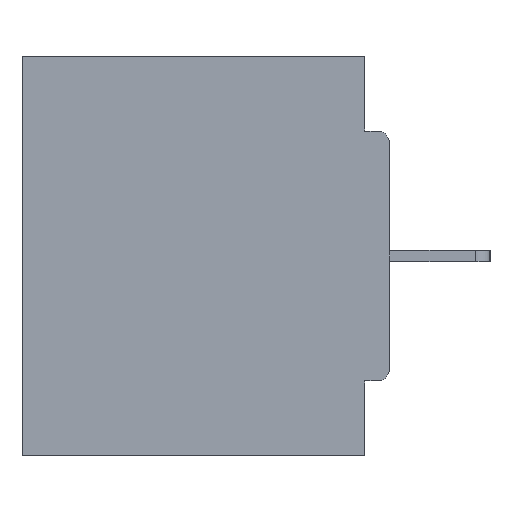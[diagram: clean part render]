
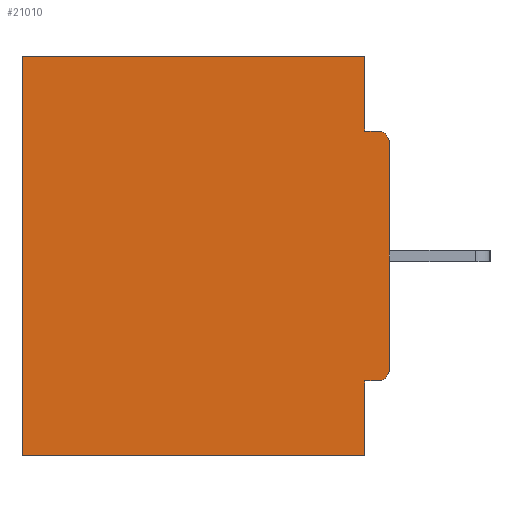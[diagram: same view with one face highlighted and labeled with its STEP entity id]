
A CAD part, left-side view. The second image highlights one B-rep face of the part: STEP entity #21010.
In plain terms, the highlighted planar face has unit normal (-1, 0, 0).
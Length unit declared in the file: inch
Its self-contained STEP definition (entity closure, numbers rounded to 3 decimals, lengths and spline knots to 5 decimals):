
#112 = VERTEX_POINT ( 'NONE', #14981 ) ;
#173 = ORIENTED_EDGE ( 'NONE', *, *, #13140, .F. ) ;
#567 = CARTESIAN_POINT ( 'NONE',  ( 0.298, 0.015, -0.0935 ) ) ;
#664 = VERTEX_POINT ( 'NONE', #13130 ) ;
#939 = EDGE_CURVE ( 'NONE', #664, #19759, #7482, .T. ) ;
#2488 = CARTESIAN_POINT ( 'NONE',  ( 0.298, 0., -0.0935 ) ) ;
#3073 = EDGE_CURVE ( 'NONE', #112, #14863, #17425, .T. ) ;
#3423 = DIRECTION ( 'NONE',  ( 0., 0., -1. ) ) ;
#4201 = VECTOR ( 'NONE', #13381, 39.37008 ) ;
#5898 = DIRECTION ( 'NONE',  ( 1., 0., 0. ) ) ;
#6306 = VERTEX_POINT ( 'NONE', #20187 ) ;
#6440 = CARTESIAN_POINT ( 'NONE',  ( 0.298, 0.015, -0.3915 ) ) ;
#6796 = DIRECTION ( 'NONE',  ( -1., 0., 0. ) ) ;
#7477 = AXIS2_PLACEMENT_3D ( 'NONE', #13451, #5898, #3423 ) ;
#7482 = LINE ( 'NONE', #27811, #12772 ) ;
#7650 = CARTESIAN_POINT ( 'NONE',  ( 0.298, 0.031, -0.5 ) ) ;
#7891 = DIRECTION ( 'NONE',  ( 0., 0., -1. ) ) ;
#8072 = LINE ( 'NONE', #2488, #15989 ) ;
#8828 = LINE ( 'NONE', #21455, #9953 ) ;
#9593 = EDGE_LOOP ( 'NONE', ( #16225, #32142, #21079, #19438, #29886, #173, #20198, #16989, #21119, #31438 ) ) ;
#9953 = VECTOR ( 'NONE', #26861, 39.37008 ) ;
#10351 = CIRCLE ( 'NONE', #22405, 0.015 ) ;
#10411 = CARTESIAN_POINT ( 'NONE',  ( 0.298, 0., 0. ) ) ;
#11147 = PLANE ( 'NONE',  #7477 ) ;
#11295 = LINE ( 'NONE', #28990, #22964 ) ;
#11372 = DIRECTION ( 'NONE',  ( -1., 0., 0. ) ) ;
#11869 = CARTESIAN_POINT ( 'NONE',  ( 0.298, 0., -0.1085 ) ) ;
#11960 = EDGE_CURVE ( 'NONE', #6306, #21548, #8828, .T. ) ;
#12712 = DIRECTION ( 'NONE',  ( 0., 0., -1. ) ) ;
#12772 = VECTOR ( 'NONE', #15191, 39.37008 ) ;
#12986 = VERTEX_POINT ( 'NONE', #7650 ) ;
#13065 = VERTEX_POINT ( 'NONE', #28127 ) ;
#13130 = CARTESIAN_POINT ( 'NONE',  ( 0.298, 0.031, 0. ) ) ;
#13140 = EDGE_CURVE ( 'NONE', #12986, #14863, #26141, .T. ) ;
#13381 = DIRECTION ( 'NONE',  ( 0., 1., 0. ) ) ;
#13451 = CARTESIAN_POINT ( 'NONE',  ( 0.298, 0., 0. ) ) ;
#13645 = LINE ( 'NONE', #28077, #25780 ) ;
#14366 = CARTESIAN_POINT ( 'NONE',  ( 0.298, 0.031, -0.4065 ) ) ;
#14863 = VERTEX_POINT ( 'NONE', #18270 ) ;
#14981 = CARTESIAN_POINT ( 'NONE',  ( 0.298, 0.46, 0. ) ) ;
#15191 = DIRECTION ( 'NONE',  ( 0., 0., -1. ) ) ;
#15989 = VECTOR ( 'NONE', #22844, 39.37008 ) ;
#16216 = DIRECTION ( 'NONE',  ( 0., 1., 0. ) ) ;
#16225 = ORIENTED_EDGE ( 'NONE', *, *, #29226, .T. ) ;
#16989 = ORIENTED_EDGE ( 'NONE', *, *, #11960, .F. ) ;
#17106 = AXIS2_PLACEMENT_3D ( 'NONE', #6440, #11372, #21368 ) ;
#17425 = LINE ( 'NONE', #27250, #18306 ) ;
#18270 = CARTESIAN_POINT ( 'NONE',  ( 0.298, 0.46, -0.5 ) ) ;
#18306 = VECTOR ( 'NONE', #7891, 39.37008 ) ;
#18346 = DIRECTION ( 'NONE',  ( 0., 0., -1. ) ) ;
#18780 = CARTESIAN_POINT ( 'NONE',  ( 0.298, 0., -0.5 ) ) ;
#19438 = ORIENTED_EDGE ( 'NONE', *, *, #31608, .T. ) ;
#19759 = VERTEX_POINT ( 'NONE', #29780 ) ;
#20187 = CARTESIAN_POINT ( 'NONE',  ( 0.298, 0.015, -0.4065 ) ) ;
#20198 = ORIENTED_EDGE ( 'NONE', *, *, #20636, .F. ) ;
#20636 = EDGE_CURVE ( 'NONE', #21548, #12986, #13645, .T. ) ;
#20678 = FACE_OUTER_BOUND ( 'NONE', #9593, .T. ) ;
#21010 = ADVANCED_FACE ( 'NONE', ( #20678 ), #11147, .F. ) ;
#21079 = ORIENTED_EDGE ( 'NONE', *, *, #939, .F. ) ;
#21119 = ORIENTED_EDGE ( 'NONE', *, *, #25135, .T. ) ;
#21368 = DIRECTION ( 'NONE',  ( 0., 0., -1. ) ) ;
#21455 = CARTESIAN_POINT ( 'NONE',  ( 0.298, 0., -0.4065 ) ) ;
#21548 = VERTEX_POINT ( 'NONE', #14366 ) ;
#21701 = VECTOR ( 'NONE', #12712, 39.37008 ) ;
#21885 = CARTESIAN_POINT ( 'NONE',  ( 0.298, 0.015, -0.1085 ) ) ;
#22078 = VERTEX_POINT ( 'NONE', #11869 ) ;
#22333 = CIRCLE ( 'NONE', #17106, 0.015 ) ;
#22405 = AXIS2_PLACEMENT_3D ( 'NONE', #21885, #6796, #18346 ) ;
#22844 = DIRECTION ( 'NONE',  ( 0., -1., 0. ) ) ;
#22964 = VECTOR ( 'NONE', #16216, 39.37008 ) ;
#23172 = DIRECTION ( 'NONE',  ( 0., 0., -1. ) ) ;
#25135 = EDGE_CURVE ( 'NONE', #6306, #13065, #22333, .T. ) ;
#25780 = VECTOR ( 'NONE', #23172, 39.37008 ) ;
#26141 = LINE ( 'NONE', #18780, #4201 ) ;
#26163 = EDGE_CURVE ( 'NONE', #22078, #13065, #30737, .T. ) ;
#26564 = EDGE_CURVE ( 'NONE', #19759, #27559, #8072, .T. ) ;
#26861 = DIRECTION ( 'NONE',  ( 0., 1., 0. ) ) ;
#27250 = CARTESIAN_POINT ( 'NONE',  ( 0.298, 0.46, 0. ) ) ;
#27559 = VERTEX_POINT ( 'NONE', #567 ) ;
#27811 = CARTESIAN_POINT ( 'NONE',  ( 0.298, 0.031, -0.5 ) ) ;
#28077 = CARTESIAN_POINT ( 'NONE',  ( 0.298, 0.031, -0.5 ) ) ;
#28127 = CARTESIAN_POINT ( 'NONE',  ( 0.298, 0., -0.3915 ) ) ;
#28990 = CARTESIAN_POINT ( 'NONE',  ( 0.298, 0., 0. ) ) ;
#29226 = EDGE_CURVE ( 'NONE', #22078, #27559, #10351, .T. ) ;
#29780 = CARTESIAN_POINT ( 'NONE',  ( 0.298, 0.031, -0.0935 ) ) ;
#29886 = ORIENTED_EDGE ( 'NONE', *, *, #3073, .T. ) ;
#30737 = LINE ( 'NONE', #10411, #21701 ) ;
#31438 = ORIENTED_EDGE ( 'NONE', *, *, #26163, .F. ) ;
#31608 = EDGE_CURVE ( 'NONE', #664, #112, #11295, .T. ) ;
#32142 = ORIENTED_EDGE ( 'NONE', *, *, #26564, .F. ) ;
